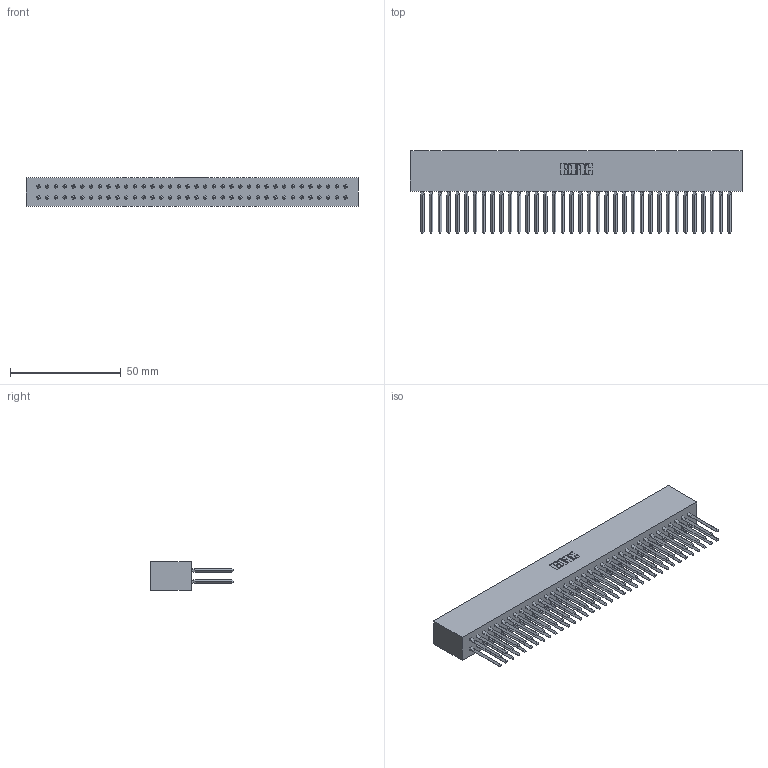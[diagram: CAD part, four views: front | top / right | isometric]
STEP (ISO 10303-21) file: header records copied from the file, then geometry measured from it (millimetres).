
FILE_DESCRIPTION (( 'STEP AP203' ), '1' );
FILE_NAME ('317-072-540-801.STEP', '2020-02-28T07:21:05', ( '' ), ( '' ), 'SwSTEP 2.0', 'SolidWorks 2016', '' );
FILE_SCHEMA (( 'CONFIG_CONTROL_DESIGN' ));
Length unit declared in the file: inch
Products named in the file (3): 317-072-540-801; 317-290-001_540; 317 Part_Lugless
Assembly tree (73 placements, depth 2):
  317-072-540-801
    317 Part_Lugless
    317-290-001_540  x72
Bounding box: 149.86 x 37.34 x 12.7 mm (x, y, z)
Volume: 26741.9 mm3; surface area: 39899.9 mm2
Topology: 73 solids, 73 shells, 6498 faces, 18023 edges, 11606 vertices
Faces by surface type: plane 5306, cylinder 904, bspline 288
Entity records: 52466 total; most frequent: CARTESIAN_POINT 9567, ORIENTED_EDGE 9066, DIRECTION 7555, EDGE_CURVE 4533, LINE 4285, VECTOR 4285, VERTEX_POINT 3015, AXIS2_PLACEMENT_3D 1635
